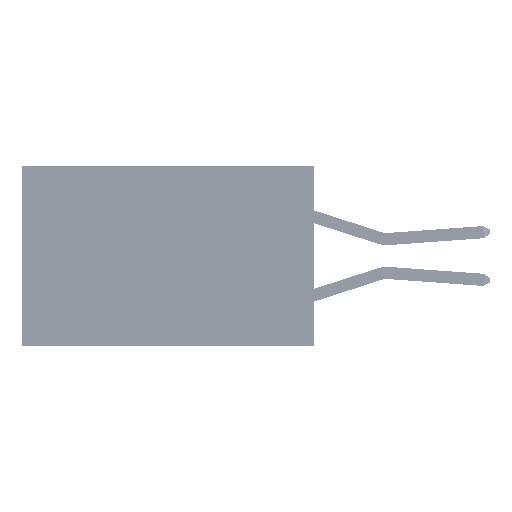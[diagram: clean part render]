
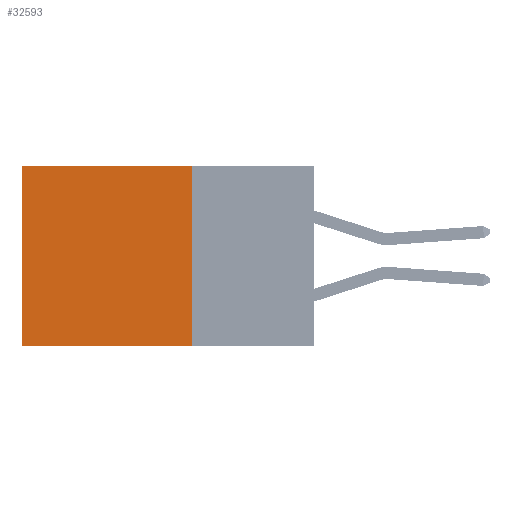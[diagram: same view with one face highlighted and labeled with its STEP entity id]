
A CAD part, left-side view. The second image highlights one B-rep face of the part: STEP entity #32593.
In plain terms, the highlighted planar face has unit normal (-1, 0, 0).
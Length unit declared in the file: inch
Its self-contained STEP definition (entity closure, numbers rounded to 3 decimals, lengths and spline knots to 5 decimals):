
#68 = VERTEX_POINT ( 'NONE', #37794 ) ;
#1516 = VECTOR ( 'NONE', #23802, 39.37008 ) ;
#3647 = CARTESIAN_POINT ( 'NONE',  ( 0.2875, 0.25, 0. ) ) ;
#4205 = VECTOR ( 'NONE', #19105, 39.37008 ) ;
#6058 = CARTESIAN_POINT ( 'NONE',  ( 0.2875, 0.6, 0. ) ) ;
#6187 = VERTEX_POINT ( 'NONE', #3647 ) ;
#6615 = CARTESIAN_POINT ( 'NONE',  ( 0.2875, 0.25, -0.37 ) ) ;
#9949 = EDGE_CURVE ( 'NONE', #6187, #20498, #35711, .T. ) ;
#9967 = DIRECTION ( 'NONE',  ( 0., 1., 0. ) ) ;
#10723 = CARTESIAN_POINT ( 'NONE',  ( 0.2875, 0.25, 0. ) ) ;
#13598 = ORIENTED_EDGE ( 'NONE', *, *, #19353, .F. ) ;
#14123 = EDGE_LOOP ( 'NONE', ( #40703, #13598, #48113, #28578 ) ) ;
#14557 = DIRECTION ( 'NONE',  ( 0., 0., -1. ) ) ;
#16657 = VECTOR ( 'NONE', #25512, 39.37008 ) ;
#17648 = VECTOR ( 'NONE', #9967, 39.37008 ) ;
#19073 = FACE_OUTER_BOUND ( 'NONE', #14123, .T. ) ;
#19105 = DIRECTION ( 'NONE',  ( 0., 0., -1. ) ) ;
#19353 = EDGE_CURVE ( 'NONE', #20498, #68, #20239, .T. ) ;
#19952 = VERTEX_POINT ( 'NONE', #6058 ) ;
#20239 = LINE ( 'NONE', #6615, #16657 ) ;
#20498 = VERTEX_POINT ( 'NONE', #24265 ) ;
#23802 = DIRECTION ( 'NONE',  ( 0., 0., -1. ) ) ;
#24265 = CARTESIAN_POINT ( 'NONE',  ( 0.2875, 0.25, -0.37 ) ) ;
#25512 = DIRECTION ( 'NONE',  ( 0., 1., 0. ) ) ;
#28578 = ORIENTED_EDGE ( 'NONE', *, *, #42048, .T. ) ;
#29642 = PLANE ( 'NONE',  #43042 ) ;
#32593 = ADVANCED_FACE ( 'NONE', ( #19073 ), #29642, .F. ) ;
#35711 = LINE ( 'NONE', #38006, #4205 ) ;
#37278 = DIRECTION ( 'NONE',  ( 1., 0., 0. ) ) ;
#37794 = CARTESIAN_POINT ( 'NONE',  ( 0.2875, 0.6, -0.37 ) ) ;
#38006 = CARTESIAN_POINT ( 'NONE',  ( 0.2875, 0.25, 0. ) ) ;
#39006 = EDGE_CURVE ( 'NONE', #19952, #68, #41886, .T. ) ;
#40360 = CARTESIAN_POINT ( 'NONE',  ( 0.2875, 0.25, 0. ) ) ;
#40703 = ORIENTED_EDGE ( 'NONE', *, *, #39006, .T. ) ;
#41886 = LINE ( 'NONE', #42735, #1516 ) ;
#42048 = EDGE_CURVE ( 'NONE', #6187, #19952, #49144, .T. ) ;
#42735 = CARTESIAN_POINT ( 'NONE',  ( 0.2875, 0.6, 0. ) ) ;
#43042 = AXIS2_PLACEMENT_3D ( 'NONE', #10723, #37278, #14557 ) ;
#48113 = ORIENTED_EDGE ( 'NONE', *, *, #9949, .F. ) ;
#49144 = LINE ( 'NONE', #40360, #17648 ) ;
